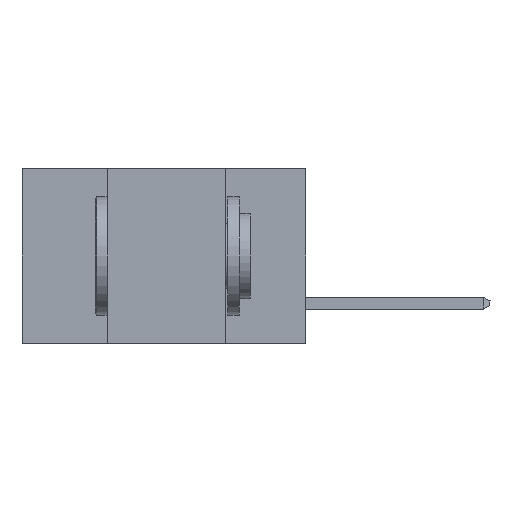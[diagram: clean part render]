
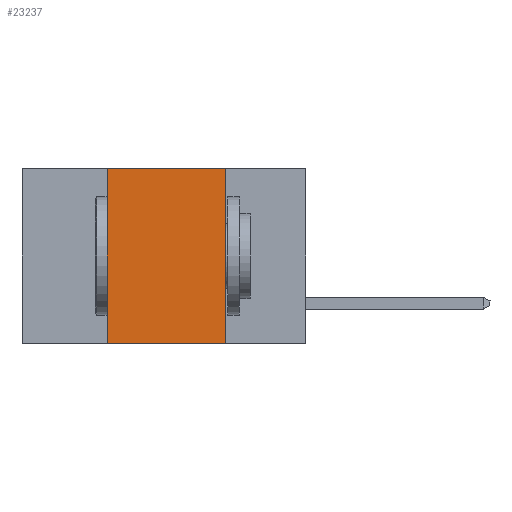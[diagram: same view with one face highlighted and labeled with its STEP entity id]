
A CAD part, left-side view. The second image highlights one B-rep face of the part: STEP entity #23237.
In plain terms, the highlighted planar face has unit normal (-1, 0, 0).
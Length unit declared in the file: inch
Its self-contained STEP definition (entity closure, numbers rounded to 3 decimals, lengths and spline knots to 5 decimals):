
#9 = CARTESIAN_POINT ( 'NONE',  ( 0., 0.6, 0. ) ) ;
#56 = CARTESIAN_POINT ( 'NONE',  ( 0., 0.17, 0. ) ) ;
#93 = EDGE_CURVE ( 'NONE', #10870, #22470, #4957, .T. ) ;
#111 = VECTOR ( 'NONE', #18146, 39.37008 ) ;
#326 = LINE ( 'NONE', #11876, #24652 ) ;
#2076 = EDGE_CURVE ( 'NONE', #9914, #22470, #326, .T. ) ;
#2088 = ORIENTED_EDGE ( 'NONE', *, *, #93, .F. ) ;
#3034 = DIRECTION ( 'NONE',  ( 0., 0., -1. ) ) ;
#3818 = LINE ( 'NONE', #17125, #18557 ) ;
#4605 = CARTESIAN_POINT ( 'NONE',  ( 0., 0.42, -0.37 ) ) ;
#4957 = LINE ( 'NONE', #6869, #10451 ) ;
#6869 = CARTESIAN_POINT ( 'NONE',  ( 0., 0.17, -0.37 ) ) ;
#7081 = CARTESIAN_POINT ( 'NONE',  ( 0., 0.42, 0. ) ) ;
#7764 = FACE_OUTER_BOUND ( 'NONE', #9855, .T. ) ;
#9855 = EDGE_LOOP ( 'NONE', ( #2088, #22347, #21442, #12676 ) ) ;
#9914 = VERTEX_POINT ( 'NONE', #23530 ) ;
#10451 = VECTOR ( 'NONE', #3034, 39.37008 ) ;
#10686 = LINE ( 'NONE', #4605, #111 ) ;
#10870 = VERTEX_POINT ( 'NONE', #56 ) ;
#11876 = CARTESIAN_POINT ( 'NONE',  ( 0., 0.6, -0.37 ) ) ;
#12676 = ORIENTED_EDGE ( 'NONE', *, *, #2076, .T. ) ;
#13323 = DIRECTION ( 'NONE',  ( 0., -1., 0. ) ) ;
#13420 = VERTEX_POINT ( 'NONE', #7081 ) ;
#13891 = DIRECTION ( 'NONE',  ( 0., -1., 0. ) ) ;
#15229 = DIRECTION ( 'NONE',  ( 1., 0., 0. ) ) ;
#16909 = CARTESIAN_POINT ( 'NONE',  ( 0., 0.17, -0.37 ) ) ;
#17125 = CARTESIAN_POINT ( 'NONE',  ( 0., 0.6, 0. ) ) ;
#18146 = DIRECTION ( 'NONE',  ( 0., 0., 1. ) ) ;
#18344 = AXIS2_PLACEMENT_3D ( 'NONE', #9, #15229, #22956 ) ;
#18557 = VECTOR ( 'NONE', #13323, 39.37008 ) ;
#19683 = EDGE_CURVE ( 'NONE', #13420, #10870, #3818, .T. ) ;
#21442 = ORIENTED_EDGE ( 'NONE', *, *, #21924, .F. ) ;
#21924 = EDGE_CURVE ( 'NONE', #9914, #13420, #10686, .T. ) ;
#22347 = ORIENTED_EDGE ( 'NONE', *, *, #19683, .F. ) ;
#22470 = VERTEX_POINT ( 'NONE', #16909 ) ;
#22956 = DIRECTION ( 'NONE',  ( 0., 0., -1. ) ) ;
#23237 = ADVANCED_FACE ( 'NONE', ( #7764 ), #24855, .F. ) ;
#23530 = CARTESIAN_POINT ( 'NONE',  ( 0., 0.42, -0.37 ) ) ;
#24652 = VECTOR ( 'NONE', #13891, 39.37008 ) ;
#24855 = PLANE ( 'NONE',  #18344 ) ;
